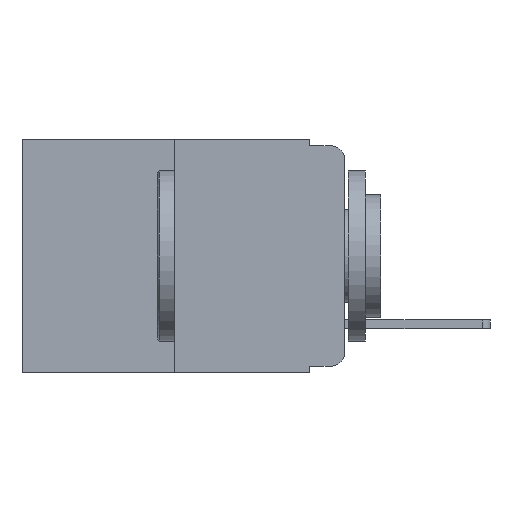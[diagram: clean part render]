
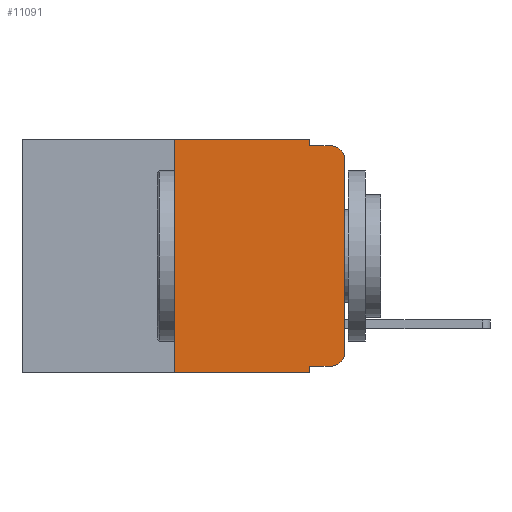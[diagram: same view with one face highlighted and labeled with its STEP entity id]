
A CAD part, left-side view. The second image highlights one B-rep face of the part: STEP entity #11091.
In plain terms, the highlighted planar face has unit normal (-1, 0, 0).
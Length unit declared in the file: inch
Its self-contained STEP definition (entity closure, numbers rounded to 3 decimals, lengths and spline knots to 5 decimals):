
#101 = AXIS2_PLACEMENT_3D ( 'NONE', #10230, #477, #11711 ) ;
#273 = CARTESIAN_POINT ( 'NONE',  ( 0., 0., -0.313 ) ) ;
#414 = ORIENTED_EDGE ( 'NONE', *, *, #10432, .T. ) ;
#477 = DIRECTION ( 'NONE',  ( -1., 0., 0. ) ) ;
#1389 = DIRECTION ( 'NONE',  ( 0., 0., 1. ) ) ;
#1432 = DIRECTION ( 'NONE',  ( 0., -1., 0. ) ) ;
#1663 = CARTESIAN_POINT ( 'NONE',  ( 0., 0.051, -0.333 ) ) ;
#1739 = VECTOR ( 'NONE', #1389, 39.37008 ) ;
#2034 = CARTESIAN_POINT ( 'NONE',  ( 0., 0.051, 0. ) ) ;
#2304 = LINE ( 'NONE', #10956, #1739 ) ;
#2377 = DIRECTION ( 'NONE',  ( -1., 0., 0. ) ) ;
#3207 = ORIENTED_EDGE ( 'NONE', *, *, #17866, .T. ) ;
#3451 = CIRCLE ( 'NONE', #101, 0.02 ) ;
#3505 = VECTOR ( 'NONE', #1432, 39.37008 ) ;
#3962 = CARTESIAN_POINT ( 'NONE',  ( 0., 0.051, -0.01 ) ) ;
#4263 = CARTESIAN_POINT ( 'NONE',  ( 0., 0.051, -0.343 ) ) ;
#4340 = LINE ( 'NONE', #16554, #19371 ) ;
#5170 = VERTEX_POINT ( 'NONE', #16126 ) ;
#5171 = DIRECTION ( 'NONE',  ( 0., 0., 1. ) ) ;
#5884 = VERTEX_POINT ( 'NONE', #8996 ) ;
#5931 = CARTESIAN_POINT ( 'NONE',  ( 0., 0.25, 0. ) ) ;
#6350 = CARTESIAN_POINT ( 'NONE',  ( 0., 0.473, -0.343 ) ) ;
#7039 = LINE ( 'NONE', #9113, #18882 ) ;
#7724 = LINE ( 'NONE', #6350, #3505 ) ;
#7790 = PLANE ( 'NONE',  #14662 ) ;
#7838 = VERTEX_POINT ( 'NONE', #1663 ) ;
#7903 = ORIENTED_EDGE ( 'NONE', *, *, #14359, .F. ) ;
#8044 = DIRECTION ( 'NONE',  ( 0., -1., 0. ) ) ;
#8215 = CARTESIAN_POINT ( 'NONE',  ( 0., 0.25, -0.343 ) ) ;
#8422 = EDGE_LOOP ( 'NONE', ( #18238, #19172, #7903, #14678, #16429, #11684, #3207, #13793, #414, #10385 ) ) ;
#8747 = DIRECTION ( 'NONE',  ( 0., 0., -1. ) ) ;
#8996 = CARTESIAN_POINT ( 'NONE',  ( 0., 0., -0.03 ) ) ;
#9093 = VERTEX_POINT ( 'NONE', #3962 ) ;
#9113 = CARTESIAN_POINT ( 'NONE',  ( 0., 0.051, 0. ) ) ;
#9282 = DIRECTION ( 'NONE',  ( 0., -1., 0. ) ) ;
#9396 = DIRECTION ( 'NONE',  ( 0., 0., -1. ) ) ;
#9451 = EDGE_CURVE ( 'NONE', #9768, #12026, #13547, .T. ) ;
#9768 = VERTEX_POINT ( 'NONE', #19515 ) ;
#10230 = CARTESIAN_POINT ( 'NONE',  ( 0., 0.02, -0.03 ) ) ;
#10385 = ORIENTED_EDGE ( 'NONE', *, *, #9451, .T. ) ;
#10432 = EDGE_CURVE ( 'NONE', #7838, #9768, #14680, .T. ) ;
#10800 = LINE ( 'NONE', #15746, #13787 ) ;
#10956 = CARTESIAN_POINT ( 'NONE',  ( 0., 0.25, 0. ) ) ;
#11034 = DIRECTION ( 'NONE',  ( 0., -1., 0. ) ) ;
#11091 = ADVANCED_FACE ( 'NONE', ( #11904 ), #7790, .F. ) ;
#11300 = VERTEX_POINT ( 'NONE', #8215 ) ;
#11305 = VECTOR ( 'NONE', #8044, 39.37008 ) ;
#11424 = EDGE_CURVE ( 'NONE', #7838, #17221, #18011, .T. ) ;
#11684 = ORIENTED_EDGE ( 'NONE', *, *, #12434, .F. ) ;
#11711 = DIRECTION ( 'NONE',  ( 0., 0., -1. ) ) ;
#11764 = CARTESIAN_POINT ( 'NONE',  ( 0., 0.02, -0.313 ) ) ;
#11904 = FACE_OUTER_BOUND ( 'NONE', #8422, .T. ) ;
#12026 = VERTEX_POINT ( 'NONE', #273 ) ;
#12233 = LINE ( 'NONE', #15446, #11305 ) ;
#12307 = EDGE_CURVE ( 'NONE', #12804, #16959, #4340, .T. ) ;
#12308 = CARTESIAN_POINT ( 'NONE',  ( 0., 0.473, 0. ) ) ;
#12434 = EDGE_CURVE ( 'NONE', #11300, #12804, #2304, .T. ) ;
#12804 = VERTEX_POINT ( 'NONE', #5931 ) ;
#13253 = DIRECTION ( 'NONE',  ( 0., 0., -1. ) ) ;
#13396 = EDGE_CURVE ( 'NONE', #16959, #9093, #7039, .T. ) ;
#13547 = CIRCLE ( 'NONE', #15496, 0.02 ) ;
#13787 = VECTOR ( 'NONE', #5171, 39.37008 ) ;
#13793 = ORIENTED_EDGE ( 'NONE', *, *, #11424, .F. ) ;
#14185 = VECTOR ( 'NONE', #8747, 39.37008 ) ;
#14225 = VECTOR ( 'NONE', #11034, 39.37008 ) ;
#14359 = EDGE_CURVE ( 'NONE', #9093, #5170, #12233, .T. ) ;
#14629 = CARTESIAN_POINT ( 'NONE',  ( 0., 0.051, 0. ) ) ;
#14662 = AXIS2_PLACEMENT_3D ( 'NONE', #12308, #18127, #9396 ) ;
#14678 = ORIENTED_EDGE ( 'NONE', *, *, #13396, .F. ) ;
#14680 = LINE ( 'NONE', #18279, #14225 ) ;
#14973 = DIRECTION ( 'NONE',  ( 0., 0., -1. ) ) ;
#15334 = EDGE_CURVE ( 'NONE', #5884, #5170, #3451, .T. ) ;
#15446 = CARTESIAN_POINT ( 'NONE',  ( 0., 0.051, -0.01 ) ) ;
#15496 = AXIS2_PLACEMENT_3D ( 'NONE', #11764, #2377, #13253 ) ;
#15746 = CARTESIAN_POINT ( 'NONE',  ( 0., 0., 0. ) ) ;
#16126 = CARTESIAN_POINT ( 'NONE',  ( 0., 0.02, -0.01 ) ) ;
#16277 = EDGE_CURVE ( 'NONE', #12026, #5884, #10800, .T. ) ;
#16429 = ORIENTED_EDGE ( 'NONE', *, *, #12307, .F. ) ;
#16554 = CARTESIAN_POINT ( 'NONE',  ( 0., 0.473, 0. ) ) ;
#16959 = VERTEX_POINT ( 'NONE', #2034 ) ;
#17221 = VERTEX_POINT ( 'NONE', #4263 ) ;
#17866 = EDGE_CURVE ( 'NONE', #11300, #17221, #7724, .T. ) ;
#18011 = LINE ( 'NONE', #14629, #14185 ) ;
#18127 = DIRECTION ( 'NONE',  ( 1., 0., 0. ) ) ;
#18238 = ORIENTED_EDGE ( 'NONE', *, *, #16277, .T. ) ;
#18279 = CARTESIAN_POINT ( 'NONE',  ( 0., 0.051, -0.333 ) ) ;
#18882 = VECTOR ( 'NONE', #14973, 39.37008 ) ;
#19172 = ORIENTED_EDGE ( 'NONE', *, *, #15334, .T. ) ;
#19371 = VECTOR ( 'NONE', #9282, 39.37008 ) ;
#19515 = CARTESIAN_POINT ( 'NONE',  ( 0., 0.02, -0.333 ) ) ;
